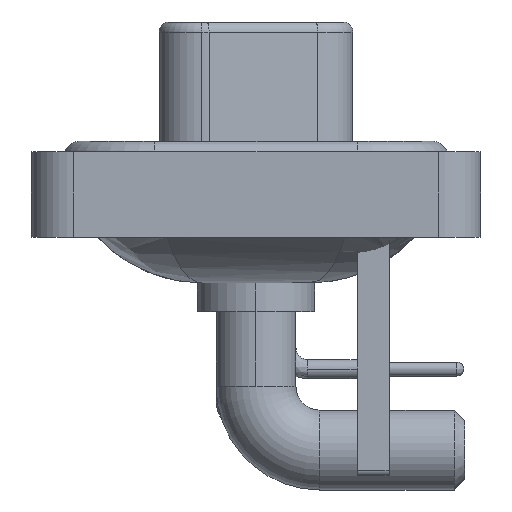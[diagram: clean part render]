
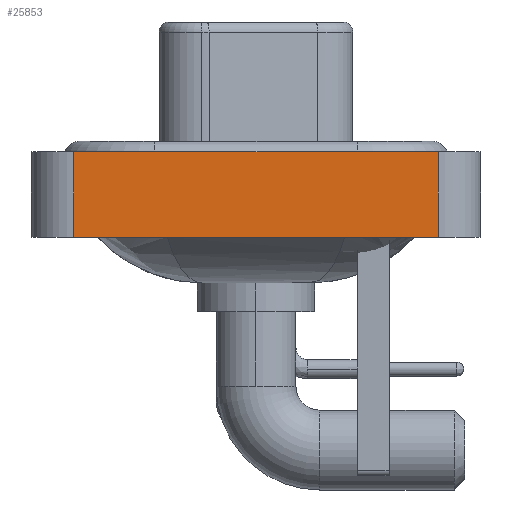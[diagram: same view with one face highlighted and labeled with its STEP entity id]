
A CAD part, left-side view. The second image highlights one B-rep face of the part: STEP entity #25853.
In plain terms, the highlighted planar face has unit normal (-1, 0, 0).
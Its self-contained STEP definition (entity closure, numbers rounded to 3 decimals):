
#368 = EDGE_CURVE ( 'NONE', #1593, #20101, #18933, .T. ) ;
#389 = FACE_OUTER_BOUND ( 'NONE', #2440, .T. ) ;
#1593 = VERTEX_POINT ( 'NONE', #18272 ) ;
#2440 = EDGE_LOOP ( 'NONE', ( #13683, #20165, #21626, #23536 ) ) ;
#3251 = CARTESIAN_POINT ( 'NONE',  ( -7.35, -8.55, -3.6 ) ) ;
#3806 = VECTOR ( 'NONE', #20933, 1000. ) ;
#3835 = AXIS2_PLACEMENT_3D ( 'NONE', #12579, #8628, #25269 ) ;
#5259 = CARTESIAN_POINT ( 'NONE',  ( -7.35, -8.55, 0.4 ) ) ;
#5546 = DIRECTION ( 'NONE',  ( 0., -1., 0. ) ) ;
#6224 = LINE ( 'NONE', #25019, #3806 ) ;
#8189 = CARTESIAN_POINT ( 'NONE',  ( -7.35, -8.55, 0.4 ) ) ;
#8628 = DIRECTION ( 'NONE',  ( -1., 0., 0. ) ) ;
#9246 = EDGE_CURVE ( 'NONE', #20101, #11033, #11365, .T. ) ;
#10513 = CARTESIAN_POINT ( 'NONE',  ( -7.35, 8.55, -3.6 ) ) ;
#11033 = VERTEX_POINT ( 'NONE', #8189 ) ;
#11365 = LINE ( 'NONE', #5259, #14235 ) ;
#12399 = DIRECTION ( 'NONE',  ( 0., 0., 1. ) ) ;
#12579 = CARTESIAN_POINT ( 'NONE',  ( -7.35, -8.55, -3.6 ) ) ;
#13227 = EDGE_CURVE ( 'NONE', #19195, #11033, #6224, .T. ) ;
#13552 = DIRECTION ( 'NONE',  ( 0., -1., 0. ) ) ;
#13683 = ORIENTED_EDGE ( 'NONE', *, *, #13227, .T. ) ;
#14235 = VECTOR ( 'NONE', #13552, 1000. ) ;
#14504 = EDGE_CURVE ( 'NONE', #1593, #19195, #26640, .T. ) ;
#15036 = CARTESIAN_POINT ( 'NONE',  ( -7.35, 8.55, 0.4 ) ) ;
#15104 = VECTOR ( 'NONE', #5546, 1000. ) ;
#15829 = CARTESIAN_POINT ( 'NONE',  ( -7.35, -8.55, -3.6 ) ) ;
#16948 = PLANE ( 'NONE',  #3835 ) ;
#18272 = CARTESIAN_POINT ( 'NONE',  ( -7.35, 8.55, -3.6 ) ) ;
#18933 = LINE ( 'NONE', #10513, #20870 ) ;
#19195 = VERTEX_POINT ( 'NONE', #15829 ) ;
#20101 = VERTEX_POINT ( 'NONE', #15036 ) ;
#20165 = ORIENTED_EDGE ( 'NONE', *, *, #9246, .F. ) ;
#20870 = VECTOR ( 'NONE', #12399, 1000. ) ;
#20933 = DIRECTION ( 'NONE',  ( 0., 0., 1. ) ) ;
#21626 = ORIENTED_EDGE ( 'NONE', *, *, #368, .F. ) ;
#23536 = ORIENTED_EDGE ( 'NONE', *, *, #14504, .T. ) ;
#25019 = CARTESIAN_POINT ( 'NONE',  ( -7.35, -8.55, -3.6 ) ) ;
#25269 = DIRECTION ( 'NONE',  ( 0., 0., 1. ) ) ;
#25853 = ADVANCED_FACE ( 'NONE', ( #389 ), #16948, .T. ) ;
#26640 = LINE ( 'NONE', #3251, #15104 ) ;
